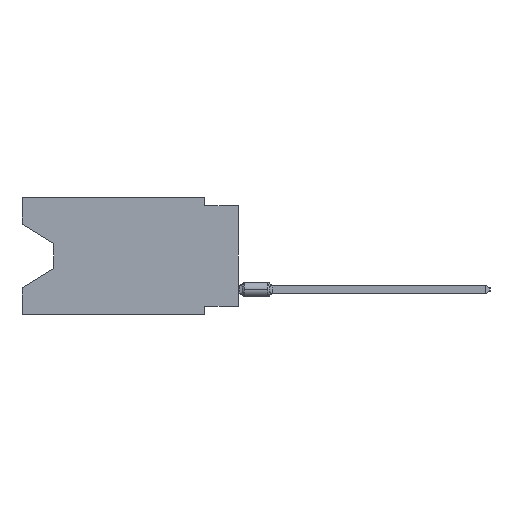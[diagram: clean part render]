
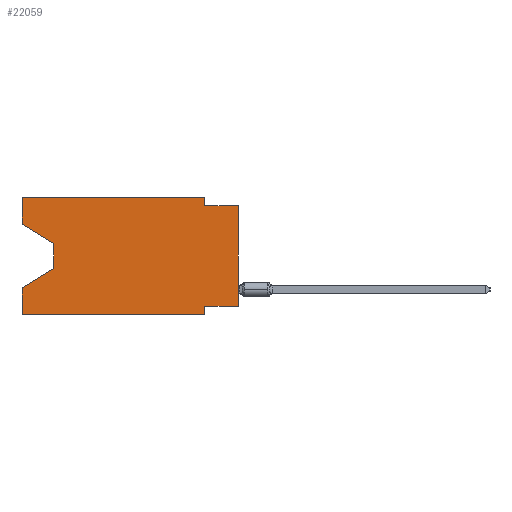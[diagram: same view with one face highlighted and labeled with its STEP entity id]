
A CAD part, left-side view. The second image highlights one B-rep face of the part: STEP entity #22059.
In plain terms, the highlighted planar face has unit normal (-1, 0, 0).
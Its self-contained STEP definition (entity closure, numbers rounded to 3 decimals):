
#322 = VECTOR ( 'NONE', #35962, 1000. ) ;
#1357 = CARTESIAN_POINT ( 'NONE',  ( 0., 13.97, -5.385 ) ) ;
#1717 = VERTEX_POINT ( 'NONE', #24431 ) ;
#2841 = VERTEX_POINT ( 'NONE', #32291 ) ;
#2986 = CARTESIAN_POINT ( 'NONE',  ( 0., 0., -8.255 ) ) ;
#3545 = DIRECTION ( 'NONE',  ( 0., 1., 0. ) ) ;
#4424 = CARTESIAN_POINT ( 'NONE',  ( 0., 16.383, 0. ) ) ;
#4890 = EDGE_CURVE ( 'NONE', #37216, #9466, #7059, .T. ) ;
#5522 = VECTOR ( 'NONE', #12569, 1000. ) ;
#6637 = CARTESIAN_POINT ( 'NONE',  ( 0., 16.383, -2.038 ) ) ;
#7059 = LINE ( 'NONE', #44001, #36857 ) ;
#7129 = EDGE_CURVE ( 'NONE', #2841, #13461, #21243, .T. ) ;
#7311 = CARTESIAN_POINT ( 'NONE',  ( 0., 2.54, 0. ) ) ;
#8931 = LINE ( 'NONE', #49674, #42523 ) ;
#9466 = VERTEX_POINT ( 'NONE', #28405 ) ;
#9878 = VERTEX_POINT ( 'NONE', #29273 ) ;
#10824 = DIRECTION ( 'NONE',  ( 1., 0., 0. ) ) ;
#10879 = CARTESIAN_POINT ( 'NONE',  ( 0., 2.54, 0. ) ) ;
#11066 = DIRECTION ( 'NONE',  ( 0., 0., 1. ) ) ;
#11279 = VECTOR ( 'NONE', #3545, 1000. ) ;
#11518 = LINE ( 'NONE', #12054, #19021 ) ;
#12039 = EDGE_CURVE ( 'NONE', #1717, #9466, #23231, .T. ) ;
#12054 = CARTESIAN_POINT ( 'NONE',  ( 0., 0., -0.635 ) ) ;
#12537 = LINE ( 'NONE', #33434, #322 ) ;
#12569 = DIRECTION ( 'NONE',  ( 0., 0., 1. ) ) ;
#12678 = ORIENTED_EDGE ( 'NONE', *, *, #12039, .T. ) ;
#13461 = VERTEX_POINT ( 'NONE', #44746 ) ;
#14087 = ORIENTED_EDGE ( 'NONE', *, *, #28896, .T. ) ;
#15034 = CARTESIAN_POINT ( 'NONE',  ( 0., 2.54, -0.635 ) ) ;
#15149 = DIRECTION ( 'NONE',  ( 0., 0., -1. ) ) ;
#15533 = CARTESIAN_POINT ( 'NONE',  ( 0., 2.54, -8.255 ) ) ;
#15662 = VERTEX_POINT ( 'NONE', #34604 ) ;
#18714 = EDGE_CURVE ( 'NONE', #2841, #9878, #24003, .T. ) ;
#19021 = VECTOR ( 'NONE', #32404, 1000. ) ;
#20923 = EDGE_CURVE ( 'NONE', #23674, #24879, #11518, .T. ) ;
#21243 = LINE ( 'NONE', #4424, #5522 ) ;
#21502 = VECTOR ( 'NONE', #37779, 1000. ) ;
#21768 = EDGE_CURVE ( 'NONE', #15662, #37216, #24452, .T. ) ;
#22059 = ADVANCED_FACE ( 'NONE', ( #48017 ), #51027, .F. ) ;
#22467 = ORIENTED_EDGE ( 'NONE', *, *, #4890, .F. ) ;
#23138 = ORIENTED_EDGE ( 'NONE', *, *, #47714, .T. ) ;
#23231 = LINE ( 'NONE', #30845, #29684 ) ;
#23674 = VERTEX_POINT ( 'NONE', #15034 ) ;
#23924 = VECTOR ( 'NONE', #33383, 1000. ) ;
#24003 = LINE ( 'NONE', #6637, #38009 ) ;
#24431 = CARTESIAN_POINT ( 'NONE',  ( 0., 16.383, -8.89 ) ) ;
#24452 = LINE ( 'NONE', #2986, #11279 ) ;
#24879 = VERTEX_POINT ( 'NONE', #50681 ) ;
#25316 = ORIENTED_EDGE ( 'NONE', *, *, #21768, .F. ) ;
#26624 = DIRECTION ( 'NONE',  ( 0., 0., -1. ) ) ;
#26921 = VERTEX_POINT ( 'NONE', #40086 ) ;
#27646 = EDGE_CURVE ( 'NONE', #48916, #23674, #27974, .T. ) ;
#27974 = LINE ( 'NONE', #7311, #37196 ) ;
#28405 = CARTESIAN_POINT ( 'NONE',  ( 0., 2.54, -8.89 ) ) ;
#28896 = EDGE_CURVE ( 'NONE', #15662, #24879, #8931, .T. ) ;
#29273 = CARTESIAN_POINT ( 'NONE',  ( 0., 13.97, -3.505 ) ) ;
#29684 = VECTOR ( 'NONE', #35183, 1000. ) ;
#30528 = ORIENTED_EDGE ( 'NONE', *, *, #40173, .F. ) ;
#30845 = CARTESIAN_POINT ( 'NONE',  ( 0., 16.383, -8.89 ) ) ;
#31691 = LINE ( 'NONE', #48247, #35834 ) ;
#32291 = CARTESIAN_POINT ( 'NONE',  ( 0., 16.383, -2.038 ) ) ;
#32314 = DIRECTION ( 'NONE',  ( 0., 0., -1. ) ) ;
#32404 = DIRECTION ( 'NONE',  ( 0., -1., 0. ) ) ;
#33023 = VERTEX_POINT ( 'NONE', #43590 ) ;
#33383 = DIRECTION ( 'NONE',  ( 0., 0., -1. ) ) ;
#33434 = CARTESIAN_POINT ( 'NONE',  ( 0., 16.383, 0. ) ) ;
#33709 = LINE ( 'NONE', #1357, #21502 ) ;
#34455 = ORIENTED_EDGE ( 'NONE', *, *, #53192, .T. ) ;
#34604 = CARTESIAN_POINT ( 'NONE',  ( 0., 0., -8.255 ) ) ;
#35183 = DIRECTION ( 'NONE',  ( 0., -1., 0. ) ) ;
#35834 = VECTOR ( 'NONE', #11066, 1000. ) ;
#35962 = DIRECTION ( 'NONE',  ( 0., -1., 0. ) ) ;
#36230 = EDGE_LOOP ( 'NONE', ( #47812, #23138, #34455, #48390, #12678, #22467, #25316, #14087, #52061, #44797, #30528, #42544 ) ) ;
#36857 = VECTOR ( 'NONE', #26624, 1000. ) ;
#37196 = VECTOR ( 'NONE', #32314, 1000. ) ;
#37216 = VERTEX_POINT ( 'NONE', #15533 ) ;
#37779 = DIRECTION ( 'NONE',  ( 0., 0.855, -0.519 ) ) ;
#38009 = VECTOR ( 'NONE', #53062, 1000. ) ;
#39913 = EDGE_CURVE ( 'NONE', #1717, #26921, #31691, .T. ) ;
#40086 = CARTESIAN_POINT ( 'NONE',  ( 0., 16.383, -6.852 ) ) ;
#40173 = EDGE_CURVE ( 'NONE', #13461, #48916, #12537, .T. ) ;
#41566 = LINE ( 'NONE', #42084, #23924 ) ;
#42084 = CARTESIAN_POINT ( 'NONE',  ( 0., 13.97, -3.505 ) ) ;
#42523 = VECTOR ( 'NONE', #53486, 1000. ) ;
#42544 = ORIENTED_EDGE ( 'NONE', *, *, #7129, .F. ) ;
#43590 = CARTESIAN_POINT ( 'NONE',  ( 0., 13.97, -5.385 ) ) ;
#44001 = CARTESIAN_POINT ( 'NONE',  ( 0., 2.54, -8.89 ) ) ;
#44234 = CARTESIAN_POINT ( 'NONE',  ( 0., 16.383, 0. ) ) ;
#44746 = CARTESIAN_POINT ( 'NONE',  ( 0., 16.383, 0. ) ) ;
#44797 = ORIENTED_EDGE ( 'NONE', *, *, #27646, .F. ) ;
#45834 = AXIS2_PLACEMENT_3D ( 'NONE', #44234, #10824, #15149 ) ;
#47714 = EDGE_CURVE ( 'NONE', #9878, #33023, #41566, .T. ) ;
#47812 = ORIENTED_EDGE ( 'NONE', *, *, #18714, .T. ) ;
#48017 = FACE_OUTER_BOUND ( 'NONE', #36230, .T. ) ;
#48247 = CARTESIAN_POINT ( 'NONE',  ( 0., 16.383, 0. ) ) ;
#48390 = ORIENTED_EDGE ( 'NONE', *, *, #39913, .F. ) ;
#48916 = VERTEX_POINT ( 'NONE', #10879 ) ;
#49674 = CARTESIAN_POINT ( 'NONE',  ( 0., 0., 0. ) ) ;
#50681 = CARTESIAN_POINT ( 'NONE',  ( 0., 0., -0.635 ) ) ;
#51027 = PLANE ( 'NONE',  #45834 ) ;
#52061 = ORIENTED_EDGE ( 'NONE', *, *, #20923, .F. ) ;
#53062 = DIRECTION ( 'NONE',  ( 0., -0.855, -0.519 ) ) ;
#53192 = EDGE_CURVE ( 'NONE', #33023, #26921, #33709, .T. ) ;
#53486 = DIRECTION ( 'NONE',  ( 0., 0., 1. ) ) ;
